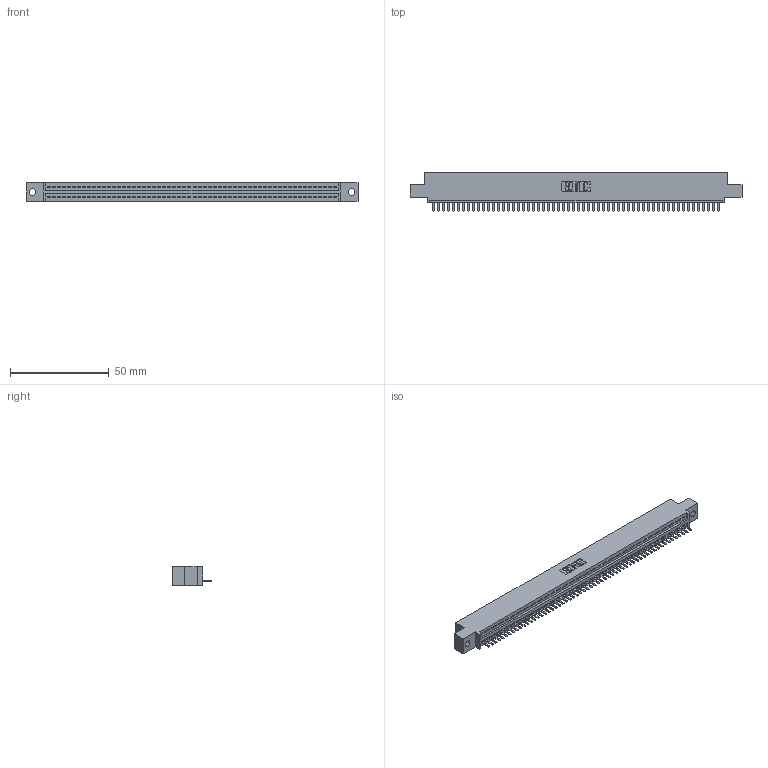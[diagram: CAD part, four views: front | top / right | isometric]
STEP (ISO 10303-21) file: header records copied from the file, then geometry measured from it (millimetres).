
FILE_DESCRIPTION (( 'STEP AP203' ), '1' );
FILE_NAME ('345-058-520-402.STEP', '2018-09-19T04:46:51', ( '' ), ( '' ), 'SwSTEP 2.0', 'SolidWorks 2016', '' );
FILE_SCHEMA (( 'CONFIG_CONTROL_DESIGN' ));
Length unit declared in the file: inch
Products named in the file (3): 345-292-001_345-293-120; 345-058-520-402; 345 Part_0.110 Offset - 0.128 Dia
Assembly tree (59 placements, depth 2):
  345-058-520-402
    345 Part_0.110 Offset - 0.128 Dia
    345-292-001_345-293-120  x58
Bounding box: 168.53 x 19.68 x 9.4 mm (x, y, z)
Volume: 15861.2 mm3; surface area: 20560.2 mm2
Topology: 59 solids, 59 shells, 3726 faces, 11025 edges, 7194 vertices
Faces by surface type: plane 2520, cylinder 1206
Entity records: 41747 total; most frequent: CARTESIAN_POINT 7250, ORIENTED_EDGE 7230, DIRECTION 6295, EDGE_CURVE 3615, VECTOR 3247, LINE 3247, VERTEX_POINT 2406, AXIS2_PLACEMENT_3D 1524
